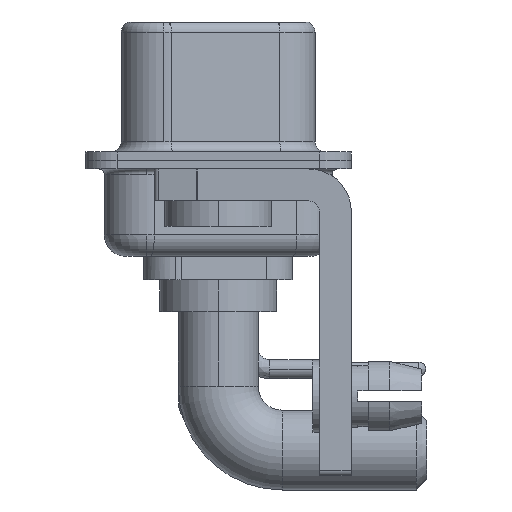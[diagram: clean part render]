
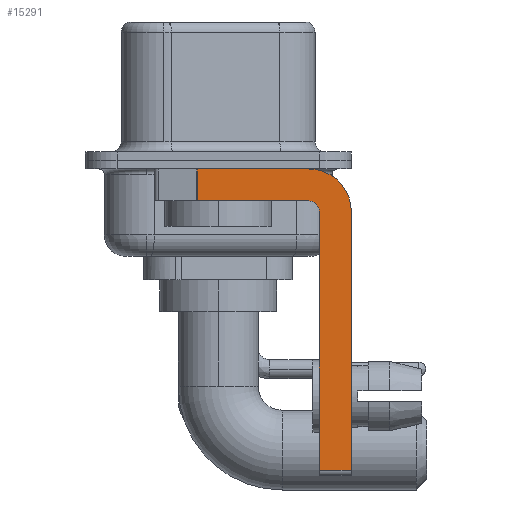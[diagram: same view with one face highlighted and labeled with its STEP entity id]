
A CAD part, left-side view. The second image highlights one B-rep face of the part: STEP entity #15291.
In plain terms, the highlighted planar face has unit normal (-1, 0, 0).
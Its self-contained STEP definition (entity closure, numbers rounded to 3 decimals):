
#40 = VECTOR ( 'NONE', #11796, 1000. ) ;
#123 = VECTOR ( 'NONE', #26802, 1000. ) ;
#161 = VECTOR ( 'NONE', #15341, 1000. ) ;
#605 = DIRECTION ( 'NONE',  ( -1., 0., 0. ) ) ;
#1411 = CARTESIAN_POINT ( 'NONE',  ( -2.9, 3., -0.4 ) ) ;
#1745 = DIRECTION ( 'NONE',  ( 0., 0., 1. ) ) ;
#2382 = DIRECTION ( 'NONE',  ( 0., 0., 1. ) ) ;
#2636 = VECTOR ( 'NONE', #17511, 1000. ) ;
#2983 = ORIENTED_EDGE ( 'NONE', *, *, #23865, .T. ) ;
#3059 = EDGE_CURVE ( 'NONE', #21307, #15196, #16398, .T. ) ;
#3451 = CARTESIAN_POINT ( 'NONE',  ( -2.9, -4.75, -14.55 ) ) ;
#3524 = CARTESIAN_POINT ( 'NONE',  ( -2.9, -4.25, -14.55 ) ) ;
#3651 = EDGE_CURVE ( 'NONE', #5991, #15196, #19298, .T. ) ;
#4428 = ORIENTED_EDGE ( 'NONE', *, *, #3059, .T. ) ;
#4883 = CARTESIAN_POINT ( 'NONE',  ( -2.9, -4.25, -0.4 ) ) ;
#4911 = CARTESIAN_POINT ( 'NONE',  ( -2.9, -6.25, -2.4 ) ) ;
#5178 = FACE_OUTER_BOUND ( 'NONE', #25443, .T. ) ;
#5991 = VERTEX_POINT ( 'NONE', #11070 ) ;
#7774 = DIRECTION ( 'NONE',  ( 0., 0., -1. ) ) ;
#7996 = EDGE_CURVE ( 'NONE', #9964, #14616, #18689, .T. ) ;
#8776 = EDGE_CURVE ( 'NONE', #21307, #19160, #20129, .T. ) ;
#9675 = ORIENTED_EDGE ( 'NONE', *, *, #15415, .F. ) ;
#9964 = VERTEX_POINT ( 'NONE', #3451 ) ;
#10044 = CIRCLE ( 'NONE', #19228, 2. ) ;
#10225 = ORIENTED_EDGE ( 'NONE', *, *, #7996, .F. ) ;
#10479 = CARTESIAN_POINT ( 'NONE',  ( -2.9, 0.978, -1.9 ) ) ;
#10784 = CARTESIAN_POINT ( 'NONE',  ( -2.9, -4.25, -2.4 ) ) ;
#11021 = CIRCLE ( 'NONE', #26341, 0.5 ) ;
#11070 = CARTESIAN_POINT ( 'NONE',  ( -2.9, -4.25, -1.9 ) ) ;
#11241 = AXIS2_PLACEMENT_3D ( 'NONE', #10784, #19130, #12012 ) ;
#11317 = VECTOR ( 'NONE', #1745, 1000. ) ;
#11796 = DIRECTION ( 'NONE',  ( 0., -1., 0. ) ) ;
#12012 = DIRECTION ( 'NONE',  ( 0., 0., -1. ) ) ;
#13517 = PLANE ( 'NONE',  #11241 ) ;
#13903 = VERTEX_POINT ( 'NONE', #4911 ) ;
#14208 = CARTESIAN_POINT ( 'NONE',  ( -2.9, -6.25, -14.55 ) ) ;
#14616 = VERTEX_POINT ( 'NONE', #20432 ) ;
#15041 = CARTESIAN_POINT ( 'NONE',  ( -2.9, 0.978, -1.9 ) ) ;
#15108 = CARTESIAN_POINT ( 'NONE',  ( -2.9, -4.25, -2.4 ) ) ;
#15196 = VERTEX_POINT ( 'NONE', #15041 ) ;
#15291 = ADVANCED_FACE ( 'NONE', ( #5178 ), #13517, .F. ) ;
#15341 = DIRECTION ( 'NONE',  ( 0., 1., 0. ) ) ;
#15415 = EDGE_CURVE ( 'NONE', #13903, #20857, #18164, .T. ) ;
#16333 = DIRECTION ( 'NONE',  ( 0., 0., -1. ) ) ;
#16398 = LINE ( 'NONE', #10479, #123 ) ;
#17511 = DIRECTION ( 'NONE',  ( 0., -1., 0. ) ) ;
#17685 = EDGE_CURVE ( 'NONE', #19160, #13903, #10044, .T. ) ;
#18131 = CARTESIAN_POINT ( 'NONE',  ( -2.9, 0.978, -0.4 ) ) ;
#18164 = LINE ( 'NONE', #26525, #21302 ) ;
#18689 = LINE ( 'NONE', #20603, #11317 ) ;
#18994 = ORIENTED_EDGE ( 'NONE', *, *, #26235, .F. ) ;
#19130 = DIRECTION ( 'NONE',  ( 1., 0., 0. ) ) ;
#19160 = VERTEX_POINT ( 'NONE', #4883 ) ;
#19228 = AXIS2_PLACEMENT_3D ( 'NONE', #22748, #22472, #16333 ) ;
#19298 = LINE ( 'NONE', #25736, #161 ) ;
#20129 = LINE ( 'NONE', #1411, #40 ) ;
#20432 = CARTESIAN_POINT ( 'NONE',  ( -2.9, -4.75, -2.4 ) ) ;
#20603 = CARTESIAN_POINT ( 'NONE',  ( -2.9, -4.75, -14.8 ) ) ;
#20857 = VERTEX_POINT ( 'NONE', #14208 ) ;
#21302 = VECTOR ( 'NONE', #7774, 1000. ) ;
#21307 = VERTEX_POINT ( 'NONE', #18131 ) ;
#21956 = ORIENTED_EDGE ( 'NONE', *, *, #17685, .F. ) ;
#22472 = DIRECTION ( 'NONE',  ( 1., 0., 0. ) ) ;
#22748 = CARTESIAN_POINT ( 'NONE',  ( -2.9, -4.25, -2.4 ) ) ;
#23865 = EDGE_CURVE ( 'NONE', #9964, #20857, #24441, .T. ) ;
#24441 = LINE ( 'NONE', #3524, #2636 ) ;
#24681 = ORIENTED_EDGE ( 'NONE', *, *, #3651, .F. ) ;
#25443 = EDGE_LOOP ( 'NONE', ( #26808, #4428, #24681, #18994, #10225, #2983, #9675, #21956 ) ) ;
#25736 = CARTESIAN_POINT ( 'NONE',  ( -2.9, -4.25, -1.9 ) ) ;
#26235 = EDGE_CURVE ( 'NONE', #14616, #5991, #11021, .T. ) ;
#26341 = AXIS2_PLACEMENT_3D ( 'NONE', #15108, #605, #2382 ) ;
#26525 = CARTESIAN_POINT ( 'NONE',  ( -2.9, -6.25, -2.4 ) ) ;
#26802 = DIRECTION ( 'NONE',  ( 0., 0., -1. ) ) ;
#26808 = ORIENTED_EDGE ( 'NONE', *, *, #8776, .F. ) ;
